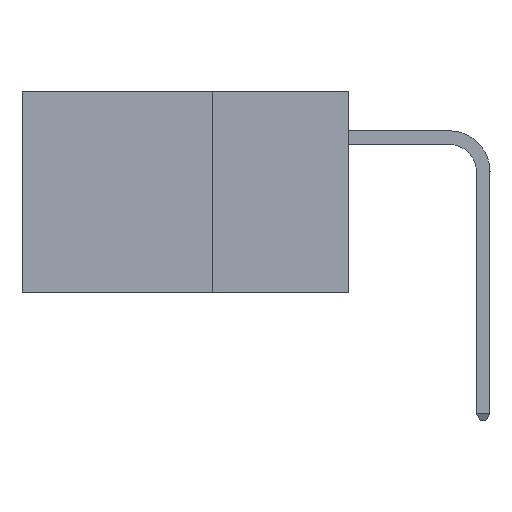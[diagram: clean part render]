
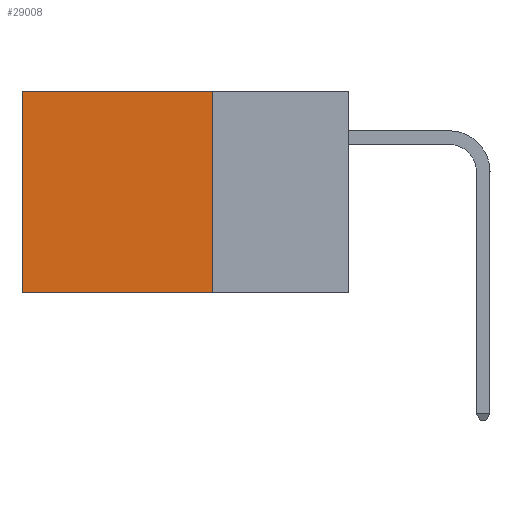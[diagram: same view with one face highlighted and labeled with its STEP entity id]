
A CAD part, left-side view. The second image highlights one B-rep face of the part: STEP entity #29008.
In plain terms, the highlighted planar face has unit normal (-1, 0, 0).
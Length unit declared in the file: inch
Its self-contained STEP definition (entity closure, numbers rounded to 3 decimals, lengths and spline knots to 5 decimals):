
#25 = VERTEX_POINT ( 'NONE', #14884 ) ;
#752 = CARTESIAN_POINT ( 'NONE',  ( 0.2875, 0.6, 0. ) ) ;
#1497 = DIRECTION ( 'NONE',  ( 1., 0., 0. ) ) ;
#3558 = VECTOR ( 'NONE', #19365, 39.37008 ) ;
#5179 = EDGE_CURVE ( 'NONE', #13439, #25, #19092, .T. ) ;
#5818 = AXIS2_PLACEMENT_3D ( 'NONE', #37503, #1497, #22686 ) ;
#6364 = DIRECTION ( 'NONE',  ( 0., 1., 0. ) ) ;
#7718 = ORIENTED_EDGE ( 'NONE', *, *, #5179, .F. ) ;
#8025 = DIRECTION ( 'NONE',  ( 0., 0., -1. ) ) ;
#9488 = VERTEX_POINT ( 'NONE', #752 ) ;
#11911 = VECTOR ( 'NONE', #8025, 39.37008 ) ;
#12257 = EDGE_CURVE ( 'NONE', #21037, #9488, #31916, .T. ) ;
#13439 = VERTEX_POINT ( 'NONE', #24084 ) ;
#14884 = CARTESIAN_POINT ( 'NONE',  ( 0.2875, 0.6, -0.37 ) ) ;
#15188 = DIRECTION ( 'NONE',  ( 0., 1., 0. ) ) ;
#16696 = PLANE ( 'NONE',  #5818 ) ;
#16779 = ORIENTED_EDGE ( 'NONE', *, *, #38376, .F. ) ;
#16813 = EDGE_LOOP ( 'NONE', ( #38088, #7718, #16779, #36560 ) ) ;
#17939 = VECTOR ( 'NONE', #15188, 39.37008 ) ;
#19092 = LINE ( 'NONE', #36804, #27005 ) ;
#19365 = DIRECTION ( 'NONE',  ( 0., 0., -1. ) ) ;
#21037 = VERTEX_POINT ( 'NONE', #33846 ) ;
#21719 = EDGE_CURVE ( 'NONE', #9488, #25, #27633, .T. ) ;
#22686 = DIRECTION ( 'NONE',  ( 0., 0., -1. ) ) ;
#24084 = CARTESIAN_POINT ( 'NONE',  ( 0.2875, 0.25, -0.37 ) ) ;
#26082 = CARTESIAN_POINT ( 'NONE',  ( 0.2875, 0.25, 0. ) ) ;
#27005 = VECTOR ( 'NONE', #6364, 39.37008 ) ;
#27633 = LINE ( 'NONE', #34194, #3558 ) ;
#27740 = FACE_OUTER_BOUND ( 'NONE', #16813, .T. ) ;
#29008 = ADVANCED_FACE ( 'NONE', ( #27740 ), #16696, .F. ) ;
#30025 = CARTESIAN_POINT ( 'NONE',  ( 0.2875, 0.25, 0. ) ) ;
#31916 = LINE ( 'NONE', #30025, #17939 ) ;
#33823 = LINE ( 'NONE', #26082, #11911 ) ;
#33846 = CARTESIAN_POINT ( 'NONE',  ( 0.2875, 0.25, 0. ) ) ;
#34194 = CARTESIAN_POINT ( 'NONE',  ( 0.2875, 0.6, 0. ) ) ;
#36560 = ORIENTED_EDGE ( 'NONE', *, *, #12257, .T. ) ;
#36804 = CARTESIAN_POINT ( 'NONE',  ( 0.2875, 0.25, -0.37 ) ) ;
#37503 = CARTESIAN_POINT ( 'NONE',  ( 0.2875, 0.25, 0. ) ) ;
#38088 = ORIENTED_EDGE ( 'NONE', *, *, #21719, .T. ) ;
#38376 = EDGE_CURVE ( 'NONE', #21037, #13439, #33823, .T. ) ;
